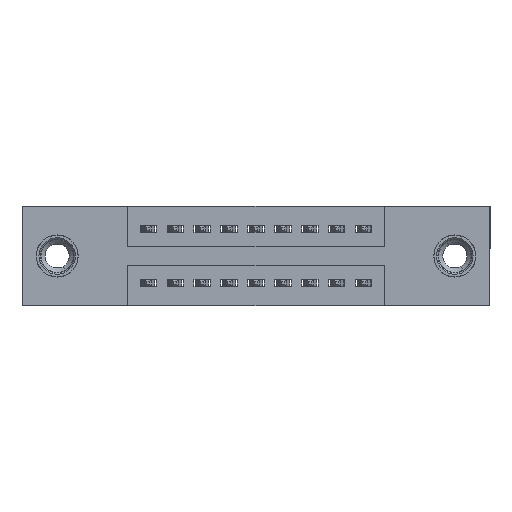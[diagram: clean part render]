
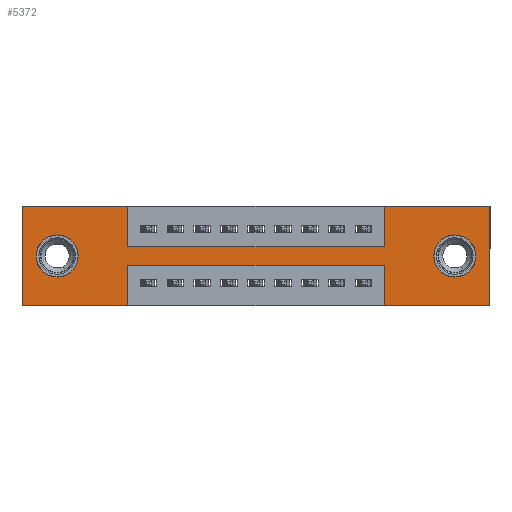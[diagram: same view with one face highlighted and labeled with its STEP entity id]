
A CAD part, front view. The second image highlights one B-rep face of the part: STEP entity #5372.
In plain terms, the highlighted planar face has unit normal (0, -1, 0).
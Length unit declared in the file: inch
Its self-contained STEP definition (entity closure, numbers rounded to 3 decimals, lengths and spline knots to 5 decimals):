
#183 = VECTOR ( 'NONE', #4214, 39.37008 ) ;
#230 = ORIENTED_EDGE ( 'NONE', *, *, #5653, .F. ) ;
#238 = CARTESIAN_POINT ( 'NONE',  ( 0.13, 0., -0.185 ) ) ;
#310 = VECTOR ( 'NONE', #10953, 39.37008 ) ;
#312 = LINE ( 'NONE', #1655, #4070 ) ;
#577 = CIRCLE ( 'NONE', #7886, 0.078 ) ;
#597 = CARTESIAN_POINT ( 'NONE',  ( 1.735, 0., -0.37 ) ) ;
#720 = VECTOR ( 'NONE', #7271, 39.37008 ) ;
#722 = DIRECTION ( 'NONE',  ( 1., 0., 0. ) ) ;
#730 = DIRECTION ( 'NONE',  ( 0., 0., -1. ) ) ;
#741 = VERTEX_POINT ( 'NONE', #4799 ) ;
#742 = EDGE_LOOP ( 'NONE', ( #13526, #12923, #4059, #13676, #9285, #230, #7521, #4309, #4552, #4470, #10285, #3720 ) ) ;
#847 = CARTESIAN_POINT ( 'NONE',  ( 0.3925, 0., -0.22 ) ) ;
#990 = EDGE_CURVE ( 'NONE', #6371, #1762, #6814, .T. ) ;
#1048 = CARTESIAN_POINT ( 'NONE',  ( 1.605, 0., -0.185 ) ) ;
#1111 = EDGE_LOOP ( 'NONE', ( #5162, #5852 ) ) ;
#1113 = DIRECTION ( 'NONE',  ( -1., 0., 0. ) ) ;
#1115 = LINE ( 'NONE', #7431, #3566 ) ;
#1147 = LINE ( 'NONE', #847, #3916 ) ;
#1158 = CARTESIAN_POINT ( 'NONE',  ( 0.13, 0., -0.107 ) ) ;
#1199 = CARTESIAN_POINT ( 'NONE',  ( 1.605, 0., -0.263 ) ) ;
#1213 = VERTEX_POINT ( 'NONE', #1199 ) ;
#1507 = VECTOR ( 'NONE', #3425, 39.37008 ) ;
#1553 = EDGE_CURVE ( 'NONE', #7068, #7583, #5953, .T. ) ;
#1587 = VERTEX_POINT ( 'NONE', #4608 ) ;
#1655 = CARTESIAN_POINT ( 'NONE',  ( 0., 0., 0. ) ) ;
#1688 = CARTESIAN_POINT ( 'NONE',  ( 0., 0., -0.37 ) ) ;
#1762 = VERTEX_POINT ( 'NONE', #3382 ) ;
#1834 = AXIS2_PLACEMENT_3D ( 'NONE', #1048, #9574, #6491 ) ;
#2069 = LINE ( 'NONE', #2144, #5678 ) ;
#2144 = CARTESIAN_POINT ( 'NONE',  ( 0.3925, 0., -0.37 ) ) ;
#2503 = CARTESIAN_POINT ( 'NONE',  ( 1.735, 0., 0. ) ) ;
#2788 = CARTESIAN_POINT ( 'NONE',  ( 1.605, 0., -0.107 ) ) ;
#2800 = CARTESIAN_POINT ( 'NONE',  ( 1.605, 0., -0.185 ) ) ;
#2890 = CARTESIAN_POINT ( 'NONE',  ( 0.3925, 0., 0. ) ) ;
#2925 = EDGE_CURVE ( 'NONE', #6769, #5046, #3138, .T. ) ;
#2929 = EDGE_LOOP ( 'NONE', ( #4911, #12301 ) ) ;
#2965 = LINE ( 'NONE', #4400, #183 ) ;
#3063 = FACE_BOUND ( 'NONE', #2929, .T. ) ;
#3138 = LINE ( 'NONE', #13645, #1507 ) ;
#3286 = CARTESIAN_POINT ( 'NONE',  ( 1.735, 0., 0. ) ) ;
#3300 = VERTEX_POINT ( 'NONE', #5120 ) ;
#3333 = VECTOR ( 'NONE', #13683, 39.37008 ) ;
#3382 = CARTESIAN_POINT ( 'NONE',  ( 0.3925, 0., -0.15 ) ) ;
#3425 = DIRECTION ( 'NONE',  ( -1., 0., 0. ) ) ;
#3456 = EDGE_CURVE ( 'NONE', #1762, #6050, #12228, .T. ) ;
#3566 = VECTOR ( 'NONE', #1113, 39.37008 ) ;
#3573 = CARTESIAN_POINT ( 'NONE',  ( 0.3925, 0., -0.15 ) ) ;
#3720 = ORIENTED_EDGE ( 'NONE', *, *, #7085, .F. ) ;
#3916 = VECTOR ( 'NONE', #8205, 39.37008 ) ;
#4028 = DIRECTION ( 'NONE',  ( 0., -1., 0. ) ) ;
#4039 = EDGE_CURVE ( 'NONE', #741, #1587, #1147, .T. ) ;
#4048 = AXIS2_PLACEMENT_3D ( 'NONE', #8318, #4028, #11566 ) ;
#4059 = ORIENTED_EDGE ( 'NONE', *, *, #10991, .F. ) ;
#4070 = VECTOR ( 'NONE', #8922, 39.37008 ) ;
#4214 = DIRECTION ( 'NONE',  ( 0., 0., 1. ) ) ;
#4226 = LINE ( 'NONE', #2503, #310 ) ;
#4309 = ORIENTED_EDGE ( 'NONE', *, *, #3456, .F. ) ;
#4400 = CARTESIAN_POINT ( 'NONE',  ( 1.3425, 0., 0. ) ) ;
#4463 = VECTOR ( 'NONE', #12317, 39.37008 ) ;
#4470 = ORIENTED_EDGE ( 'NONE', *, *, #4699, .F. ) ;
#4506 = LINE ( 'NONE', #10403, #720 ) ;
#4552 = ORIENTED_EDGE ( 'NONE', *, *, #990, .F. ) ;
#4608 = CARTESIAN_POINT ( 'NONE',  ( 0.3925, 0., -0.22 ) ) ;
#4654 = DIRECTION ( 'NONE',  ( 0., 0., 1. ) ) ;
#4699 = EDGE_CURVE ( 'NONE', #3300, #6371, #312, .T. ) ;
#4786 = VERTEX_POINT ( 'NONE', #2788 ) ;
#4799 = CARTESIAN_POINT ( 'NONE',  ( 1.3425, 0., -0.22 ) ) ;
#4911 = ORIENTED_EDGE ( 'NONE', *, *, #10767, .T. ) ;
#4925 = VECTOR ( 'NONE', #12935, 39.37008 ) ;
#5046 = VERTEX_POINT ( 'NONE', #5363 ) ;
#5120 = CARTESIAN_POINT ( 'NONE',  ( 0., 0., 0. ) ) ;
#5162 = ORIENTED_EDGE ( 'NONE', *, *, #9008, .T. ) ;
#5363 = CARTESIAN_POINT ( 'NONE',  ( 1.3425, 0., -0.37 ) ) ;
#5372 = ADVANCED_FACE ( 'NONE', ( #3063, #5718, #6376 ), #9430, .T. ) ;
#5474 = LINE ( 'NONE', #11252, #4463 ) ;
#5547 = CARTESIAN_POINT ( 'NONE',  ( 0.3925, 0., -0.37 ) ) ;
#5550 = DIRECTION ( 'NONE',  ( 0., 0., 1. ) ) ;
#5653 = EDGE_CURVE ( 'NONE', #10223, #7910, #7514, .T. ) ;
#5678 = VECTOR ( 'NONE', #7728, 39.37008 ) ;
#5718 = FACE_BOUND ( 'NONE', #1111, .T. ) ;
#5761 = VERTEX_POINT ( 'NONE', #1688 ) ;
#5852 = ORIENTED_EDGE ( 'NONE', *, *, #1553, .T. ) ;
#5953 = CIRCLE ( 'NONE', #8702, 0.078 ) ;
#6050 = VERTEX_POINT ( 'NONE', #8333 ) ;
#6371 = VERTEX_POINT ( 'NONE', #2890 ) ;
#6376 = FACE_OUTER_BOUND ( 'NONE', #742, .T. ) ;
#6491 = DIRECTION ( 'NONE',  ( 0., 0., -1. ) ) ;
#6668 = DIRECTION ( 'NONE',  ( 0., 1., 0. ) ) ;
#6769 = VERTEX_POINT ( 'NONE', #597 ) ;
#6814 = LINE ( 'NONE', #12775, #3333 ) ;
#6892 = EDGE_CURVE ( 'NONE', #7910, #6769, #4226, .T. ) ;
#7035 = CARTESIAN_POINT ( 'NONE',  ( 0., 0., 0. ) ) ;
#7068 = VERTEX_POINT ( 'NONE', #13321 ) ;
#7085 = EDGE_CURVE ( 'NONE', #9377, #5761, #1115, .T. ) ;
#7271 = DIRECTION ( 'NONE',  ( 0., 0., 1. ) ) ;
#7431 = CARTESIAN_POINT ( 'NONE',  ( 0., 0., -0.37 ) ) ;
#7514 = LINE ( 'NONE', #7035, #8843 ) ;
#7521 = ORIENTED_EDGE ( 'NONE', *, *, #12057, .F. ) ;
#7583 = VERTEX_POINT ( 'NONE', #1158 ) ;
#7728 = DIRECTION ( 'NONE',  ( 0., 0., -1. ) ) ;
#7886 = AXIS2_PLACEMENT_3D ( 'NONE', #238, #6668, #5550 ) ;
#7910 = VERTEX_POINT ( 'NONE', #3286 ) ;
#8205 = DIRECTION ( 'NONE',  ( -1., 0., 0. ) ) ;
#8318 = CARTESIAN_POINT ( 'NONE',  ( 0., 0., -0.37 ) ) ;
#8333 = CARTESIAN_POINT ( 'NONE',  ( 1.3425, 0., -0.15 ) ) ;
#8702 = AXIS2_PLACEMENT_3D ( 'NONE', #8858, #12059, #4654 ) ;
#8843 = VECTOR ( 'NONE', #722, 39.37008 ) ;
#8858 = CARTESIAN_POINT ( 'NONE',  ( 0.13, 0., -0.185 ) ) ;
#8868 = EDGE_CURVE ( 'NONE', #1587, #9377, #2069, .T. ) ;
#8922 = DIRECTION ( 'NONE',  ( 1., 0., 0. ) ) ;
#9008 = EDGE_CURVE ( 'NONE', #7583, #7068, #577, .T. ) ;
#9285 = ORIENTED_EDGE ( 'NONE', *, *, #6892, .F. ) ;
#9377 = VERTEX_POINT ( 'NONE', #5547 ) ;
#9430 = PLANE ( 'NONE',  #4048 ) ;
#9574 = DIRECTION ( 'NONE',  ( 0., 1., 0. ) ) ;
#9705 = EDGE_CURVE ( 'NONE', #5761, #3300, #4506, .T. ) ;
#9767 = CIRCLE ( 'NONE', #1834, 0.078 ) ;
#10186 = DIRECTION ( 'NONE',  ( 0., 1., 0. ) ) ;
#10223 = VERTEX_POINT ( 'NONE', #10964 ) ;
#10285 = ORIENTED_EDGE ( 'NONE', *, *, #9705, .F. ) ;
#10403 = CARTESIAN_POINT ( 'NONE',  ( 0., 0., 0. ) ) ;
#10611 = EDGE_CURVE ( 'NONE', #1213, #4786, #11276, .T. ) ;
#10767 = EDGE_CURVE ( 'NONE', #4786, #1213, #9767, .T. ) ;
#10953 = DIRECTION ( 'NONE',  ( 0., 0., -1. ) ) ;
#10964 = CARTESIAN_POINT ( 'NONE',  ( 1.3425, 0., 0. ) ) ;
#10991 = EDGE_CURVE ( 'NONE', #5046, #741, #5474, .T. ) ;
#11252 = CARTESIAN_POINT ( 'NONE',  ( 1.3425, 0., -0.37 ) ) ;
#11276 = CIRCLE ( 'NONE', #11983, 0.078 ) ;
#11566 = DIRECTION ( 'NONE',  ( 0., 0., -1. ) ) ;
#11983 = AXIS2_PLACEMENT_3D ( 'NONE', #2800, #10186, #730 ) ;
#12057 = EDGE_CURVE ( 'NONE', #6050, #10223, #2965, .T. ) ;
#12059 = DIRECTION ( 'NONE',  ( 0., 1., 0. ) ) ;
#12228 = LINE ( 'NONE', #3573, #4925 ) ;
#12301 = ORIENTED_EDGE ( 'NONE', *, *, #10611, .T. ) ;
#12317 = DIRECTION ( 'NONE',  ( 0., 0., 1. ) ) ;
#12775 = CARTESIAN_POINT ( 'NONE',  ( 0.3925, 0., 0. ) ) ;
#12923 = ORIENTED_EDGE ( 'NONE', *, *, #4039, .F. ) ;
#12935 = DIRECTION ( 'NONE',  ( 1., 0., 0. ) ) ;
#13321 = CARTESIAN_POINT ( 'NONE',  ( 0.13, 0., -0.263 ) ) ;
#13526 = ORIENTED_EDGE ( 'NONE', *, *, #8868, .F. ) ;
#13645 = CARTESIAN_POINT ( 'NONE',  ( 0., 0., -0.37 ) ) ;
#13676 = ORIENTED_EDGE ( 'NONE', *, *, #2925, .F. ) ;
#13683 = DIRECTION ( 'NONE',  ( 0., 0., -1. ) ) ;
